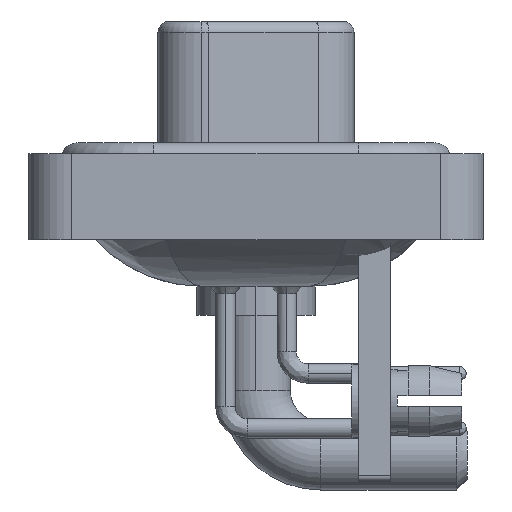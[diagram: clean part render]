
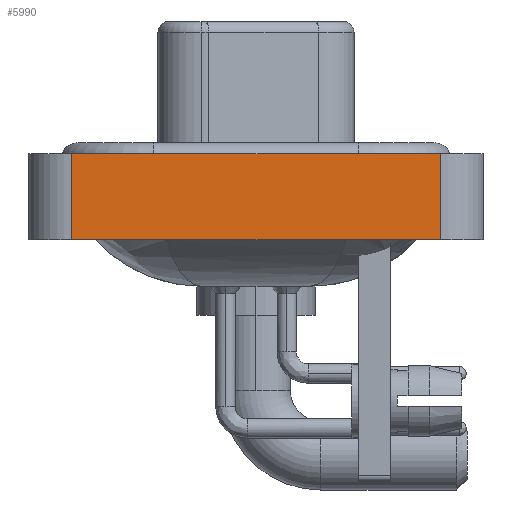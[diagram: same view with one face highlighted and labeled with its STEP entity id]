
A CAD part, left-side view. The second image highlights one B-rep face of the part: STEP entity #5990.
In plain terms, the highlighted planar face has unit normal (-1, 0, 0).
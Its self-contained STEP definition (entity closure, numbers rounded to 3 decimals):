
#717 = EDGE_CURVE ( 'NONE', #17479, #16776, #23641, .T. ) ;
#1075 = ORIENTED_EDGE ( 'NONE', *, *, #5552, .T. ) ;
#1691 = VECTOR ( 'NONE', #3674, 1000. ) ;
#1958 = EDGE_LOOP ( 'NONE', ( #29172, #26921, #11838, #1075 ) ) ;
#2243 = VERTEX_POINT ( 'NONE', #30631 ) ;
#2401 = VERTEX_POINT ( 'NONE', #4296 ) ;
#3065 = CARTESIAN_POINT ( 'NONE',  ( -7.35, -8.55, -3.6 ) ) ;
#3674 = DIRECTION ( 'NONE',  ( 0., -1., 0. ) ) ;
#3750 = DIRECTION ( 'NONE',  ( 0., 0., 1. ) ) ;
#3869 = DIRECTION ( 'NONE',  ( 0., 0., 1. ) ) ;
#4186 = AXIS2_PLACEMENT_3D ( 'NONE', #8704, #8868, #3869 ) ;
#4296 = CARTESIAN_POINT ( 'NONE',  ( -7.35, -8.55, 0.4 ) ) ;
#5552 = EDGE_CURVE ( 'NONE', #17479, #2243, #18438, .T. ) ;
#5990 = ADVANCED_FACE ( 'NONE', ( #21164 ), #26010, .T. ) ;
#8704 = CARTESIAN_POINT ( 'NONE',  ( -7.35, -8.55, -3.6 ) ) ;
#8868 = DIRECTION ( 'NONE',  ( -1., 0., 0. ) ) ;
#9841 = EDGE_CURVE ( 'NONE', #2243, #2401, #27634, .T. ) ;
#11838 = ORIENTED_EDGE ( 'NONE', *, *, #717, .F. ) ;
#12758 = EDGE_CURVE ( 'NONE', #16776, #2401, #20812, .T. ) ;
#16776 = VERTEX_POINT ( 'NONE', #26579 ) ;
#17479 = VERTEX_POINT ( 'NONE', #28582 ) ;
#18068 = VECTOR ( 'NONE', #28312, 1000. ) ;
#18438 = LINE ( 'NONE', #23779, #18068 ) ;
#20335 = VECTOR ( 'NONE', #23106, 1000. ) ;
#20812 = LINE ( 'NONE', #22910, #1691 ) ;
#20895 = CARTESIAN_POINT ( 'NONE',  ( -7.35, 8.55, -3.6 ) ) ;
#21164 = FACE_OUTER_BOUND ( 'NONE', #1958, .T. ) ;
#21829 = VECTOR ( 'NONE', #3750, 1000. ) ;
#22910 = CARTESIAN_POINT ( 'NONE',  ( -7.35, -8.55, 0.4 ) ) ;
#23106 = DIRECTION ( 'NONE',  ( 0., 0., 1. ) ) ;
#23641 = LINE ( 'NONE', #20895, #21829 ) ;
#23779 = CARTESIAN_POINT ( 'NONE',  ( -7.35, -8.55, -3.6 ) ) ;
#26010 = PLANE ( 'NONE',  #4186 ) ;
#26579 = CARTESIAN_POINT ( 'NONE',  ( -7.35, 8.55, 0.4 ) ) ;
#26921 = ORIENTED_EDGE ( 'NONE', *, *, #12758, .F. ) ;
#27634 = LINE ( 'NONE', #3065, #20335 ) ;
#28312 = DIRECTION ( 'NONE',  ( 0., -1., 0. ) ) ;
#28582 = CARTESIAN_POINT ( 'NONE',  ( -7.35, 8.55, -3.6 ) ) ;
#29172 = ORIENTED_EDGE ( 'NONE', *, *, #9841, .T. ) ;
#30631 = CARTESIAN_POINT ( 'NONE',  ( -7.35, -8.55, -3.6 ) ) ;
